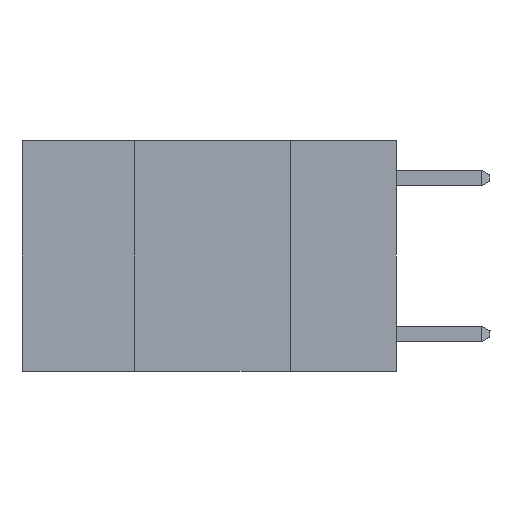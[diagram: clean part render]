
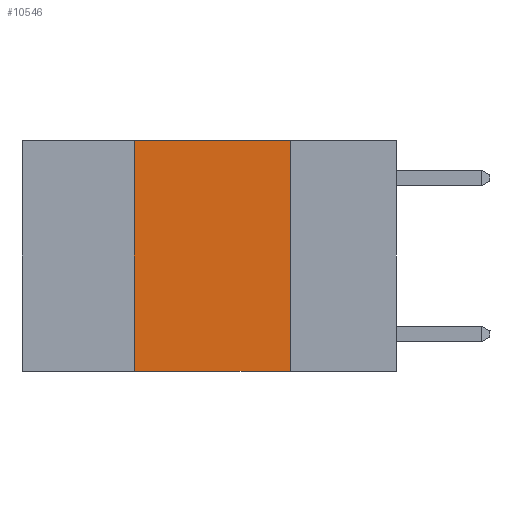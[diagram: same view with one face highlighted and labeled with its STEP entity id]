
A CAD part, left-side view. The second image highlights one B-rep face of the part: STEP entity #10546.
In plain terms, the highlighted planar face has unit normal (-1, 0, 0).
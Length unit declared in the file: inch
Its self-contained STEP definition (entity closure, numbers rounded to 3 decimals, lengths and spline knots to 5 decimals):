
#39 = VECTOR ( 'NONE', #252, 39.37008 ) ;
#162 = LINE ( 'NONE', #12347, #39 ) ;
#192 = VERTEX_POINT ( 'NONE', #13194 ) ;
#252 = DIRECTION ( 'NONE',  ( 0., 0., -1. ) ) ;
#876 = EDGE_CURVE ( 'NONE', #19960, #18830, #4822, .T. ) ;
#1444 = EDGE_CURVE ( 'NONE', #192, #19960, #20273, .T. ) ;
#1680 = CARTESIAN_POINT ( 'NONE',  ( 0., 0.17, 0. ) ) ;
#2206 = CARTESIAN_POINT ( 'NONE',  ( 0., 0.6, 0. ) ) ;
#2288 = DIRECTION ( 'NONE',  ( 1., 0., 0. ) ) ;
#2379 = AXIS2_PLACEMENT_3D ( 'NONE', #2206, #2288, #14227 ) ;
#4027 = CARTESIAN_POINT ( 'NONE',  ( 0., 0.42, 0. ) ) ;
#4822 = LINE ( 'NONE', #17085, #4877 ) ;
#4877 = VECTOR ( 'NONE', #18992, 39.37008 ) ;
#5005 = EDGE_CURVE ( 'NONE', #18830, #7100, #162, .T. ) ;
#5298 = ORIENTED_EDGE ( 'NONE', *, *, #5005, .F. ) ;
#5621 = CARTESIAN_POINT ( 'NONE',  ( 0., 0.6, -0.37 ) ) ;
#5905 = ORIENTED_EDGE ( 'NONE', *, *, #876, .F. ) ;
#6136 = ORIENTED_EDGE ( 'NONE', *, *, #1444, .F. ) ;
#6209 = ORIENTED_EDGE ( 'NONE', *, *, #21139, .T. ) ;
#7100 = VERTEX_POINT ( 'NONE', #12545 ) ;
#8582 = VECTOR ( 'NONE', #10758, 39.37008 ) ;
#8800 = EDGE_LOOP ( 'NONE', ( #5298, #5905, #6136, #6209 ) ) ;
#10546 = ADVANCED_FACE ( 'NONE', ( #13938 ), #17538, .F. ) ;
#10758 = DIRECTION ( 'NONE',  ( 0., -1., 0. ) ) ;
#12347 = CARTESIAN_POINT ( 'NONE',  ( 0., 0.17, 0. ) ) ;
#12545 = CARTESIAN_POINT ( 'NONE',  ( 0., 0.17, -0.37 ) ) ;
#13194 = CARTESIAN_POINT ( 'NONE',  ( 0., 0.42, -0.37 ) ) ;
#13938 = FACE_OUTER_BOUND ( 'NONE', #8800, .T. ) ;
#14227 = DIRECTION ( 'NONE',  ( 0., 0., -1. ) ) ;
#15832 = DIRECTION ( 'NONE',  ( 0., 0., 1. ) ) ;
#17085 = CARTESIAN_POINT ( 'NONE',  ( 0., 0.6, 0. ) ) ;
#17538 = PLANE ( 'NONE',  #2379 ) ;
#18830 = VERTEX_POINT ( 'NONE', #1680 ) ;
#18992 = DIRECTION ( 'NONE',  ( 0., -1., 0. ) ) ;
#19192 = CARTESIAN_POINT ( 'NONE',  ( 0., 0.42, 0. ) ) ;
#19960 = VERTEX_POINT ( 'NONE', #19192 ) ;
#20273 = LINE ( 'NONE', #4027, #20569 ) ;
#20569 = VECTOR ( 'NONE', #15832, 39.37008 ) ;
#21139 = EDGE_CURVE ( 'NONE', #192, #7100, #21341, .T. ) ;
#21341 = LINE ( 'NONE', #5621, #8582 ) ;
